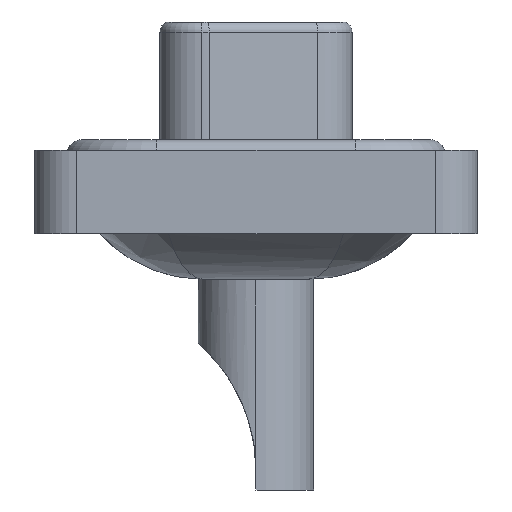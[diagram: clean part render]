
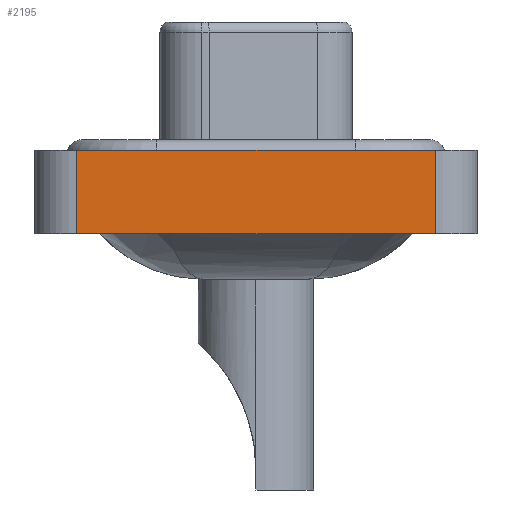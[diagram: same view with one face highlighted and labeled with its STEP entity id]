
A CAD part, left-side view. The second image highlights one B-rep face of the part: STEP entity #2195.
In plain terms, the highlighted planar face has unit normal (-1, 0, 0).
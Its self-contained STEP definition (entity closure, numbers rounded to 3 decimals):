
#16 = FACE_OUTER_BOUND ( 'NONE', #16385, .T. ) ;
#254 = EDGE_CURVE ( 'NONE', #7570, #14020, #17813, .T. ) ;
#740 = EDGE_CURVE ( 'NONE', #9372, #7570, #4024, .T. ) ;
#755 = CARTESIAN_POINT ( 'NONE',  ( -7.25, -8.55, -3.6 ) ) ;
#983 = EDGE_CURVE ( 'NONE', #3943, #14020, #7873, .T. ) ;
#1693 = CARTESIAN_POINT ( 'NONE',  ( -7.25, -8.55, 0.4 ) ) ;
#2195 = ADVANCED_FACE ( 'NONE', ( #16 ), #2932, .T. ) ;
#2343 = CARTESIAN_POINT ( 'NONE',  ( -7.25, -8.55, -3.6 ) ) ;
#2932 = PLANE ( 'NONE',  #3341 ) ;
#3307 = LINE ( 'NONE', #755, #3663 ) ;
#3341 = AXIS2_PLACEMENT_3D ( 'NONE', #4204, #15318, #8650 ) ;
#3663 = VECTOR ( 'NONE', #6018, 1000. ) ;
#3801 = DIRECTION ( 'NONE',  ( 0., 0., 1. ) ) ;
#3943 = VERTEX_POINT ( 'NONE', #12987 ) ;
#3950 = DIRECTION ( 'NONE',  ( 0., -1., 0. ) ) ;
#4024 = LINE ( 'NONE', #12385, #14318 ) ;
#4204 = CARTESIAN_POINT ( 'NONE',  ( -7.25, -8.55, -3.6 ) ) ;
#6018 = DIRECTION ( 'NONE',  ( 0., -1., 0. ) ) ;
#6517 = ORIENTED_EDGE ( 'NONE', *, *, #16526, .T. ) ;
#6810 = VECTOR ( 'NONE', #3950, 1000. ) ;
#7570 = VERTEX_POINT ( 'NONE', #16227 ) ;
#7873 = LINE ( 'NONE', #2343, #11718 ) ;
#8650 = DIRECTION ( 'NONE',  ( 0., 0., 1. ) ) ;
#9372 = VERTEX_POINT ( 'NONE', #16306 ) ;
#10542 = ORIENTED_EDGE ( 'NONE', *, *, #983, .T. ) ;
#10908 = ORIENTED_EDGE ( 'NONE', *, *, #254, .F. ) ;
#11718 = VECTOR ( 'NONE', #3801, 1000. ) ;
#12385 = CARTESIAN_POINT ( 'NONE',  ( -7.25, 8.55, -3.6 ) ) ;
#12987 = CARTESIAN_POINT ( 'NONE',  ( -7.25, -8.55, -3.6 ) ) ;
#14020 = VERTEX_POINT ( 'NONE', #1693 ) ;
#14318 = VECTOR ( 'NONE', #17792, 1000. ) ;
#14877 = CARTESIAN_POINT ( 'NONE',  ( -7.25, -8.55, 0.4 ) ) ;
#15264 = ORIENTED_EDGE ( 'NONE', *, *, #740, .F. ) ;
#15318 = DIRECTION ( 'NONE',  ( -1., 0., 0. ) ) ;
#16227 = CARTESIAN_POINT ( 'NONE',  ( -7.25, 8.55, 0.4 ) ) ;
#16306 = CARTESIAN_POINT ( 'NONE',  ( -7.25, 8.55, -3.6 ) ) ;
#16385 = EDGE_LOOP ( 'NONE', ( #10542, #10908, #15264, #6517 ) ) ;
#16526 = EDGE_CURVE ( 'NONE', #9372, #3943, #3307, .T. ) ;
#17792 = DIRECTION ( 'NONE',  ( 0., 0., 1. ) ) ;
#17813 = LINE ( 'NONE', #14877, #6810 ) ;
